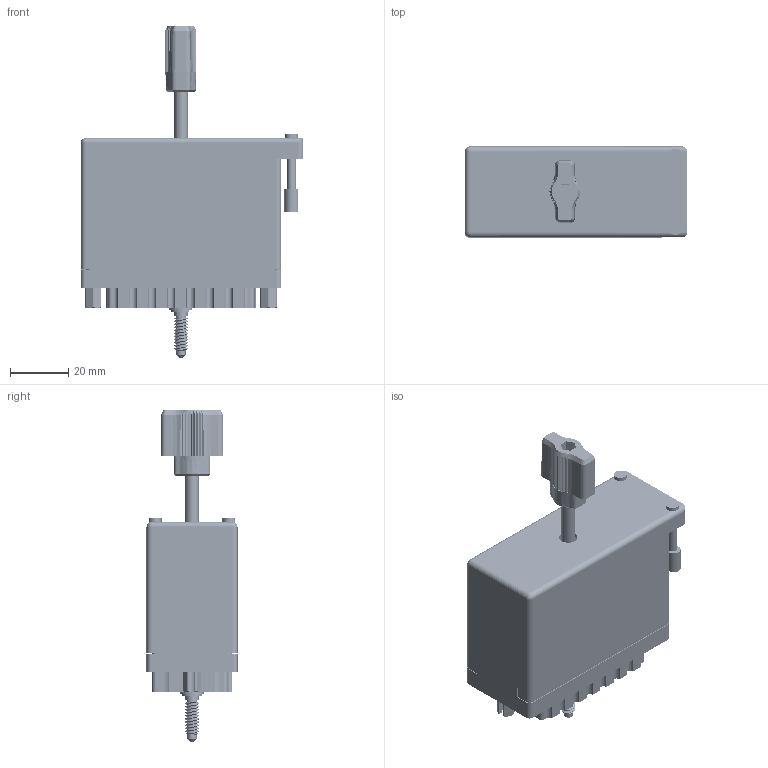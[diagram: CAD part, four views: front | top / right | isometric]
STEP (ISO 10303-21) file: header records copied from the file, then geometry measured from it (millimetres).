
FILE_DESCRIPTION (( 'STEP AP203' ), '1' );
FILE_NAME ('516-090-501-651.STEP', '2020-09-08T18:34:51', ( '' ), ( '' ), 'SwSTEP 2.0', 'SolidWorks 2020', '' );
FILE_SCHEMA (( 'CONFIG_CONTROL_DESIGN' ));
Length unit declared in the file: inch
Products named in the file (14): 516-221-090-102_090; 516-221-090-102_091; 516-230-001_Metal - 090 Side Entry; 516-253-190-107; 516-254-091-109; 516-251-095-100; 516-253-095-100; Actuating Screw Assy 090-120; 516-250-091-111; 516-090-501-651; 516 Part Receptacle_090; 516-292-001_501 Contact; Grub Screw; 516-252-091-102
Assembly tree (105 placements, depth 3):
  516-090-501-651
    516 Part Receptacle_090
    516-292-001_501 Contact  x91
    516-230-001_Metal - 090 Side Entry
    516-252-091-102  x2
    516-221-090-102_090
    Actuating Screw Assy 090-120
      516-251-095-100
      516-254-091-109
      516-253-095-100  x2
      516-253-190-107
      516-250-091-111
      Grub Screw
    516-221-090-102_091
Bounding box: 76.66 x 31.34 x 114.34 mm (x, y, z)
Volume: 43649.5 mm3; surface area: 74070.4 mm2
Topology: 104 solids, 104 shells, 8998 faces, 26001 edges, 17230 vertices
Faces by surface type: plane 5297, cylinder 3018, bspline 585, cone 96, sphere 2
Entity records: 98676 total; most frequent: CARTESIAN_POINT 27717, ORIENTED_EDGE 14370, DIRECTION 13767, EDGE_CURVE 7185, VECTOR 4935, LINE 4935, VERTEX_POINT 4750, AXIS2_PLACEMENT_3D 4416
